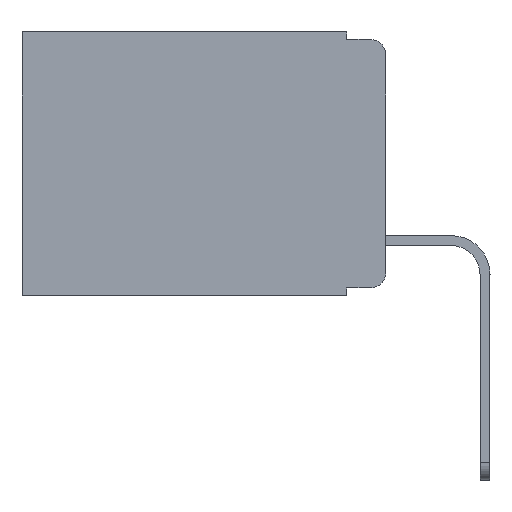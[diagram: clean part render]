
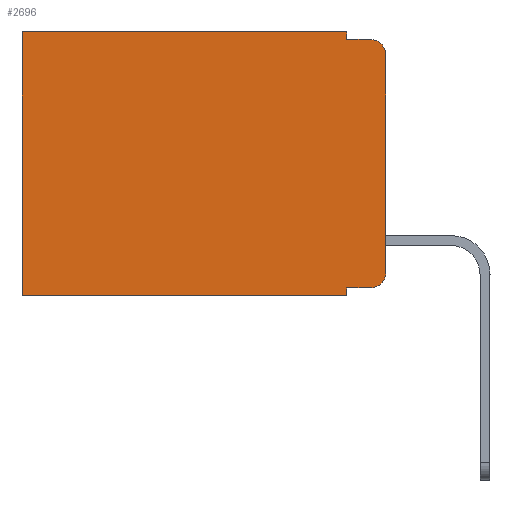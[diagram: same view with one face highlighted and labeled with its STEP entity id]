
A CAD part, left-side view. The second image highlights one B-rep face of the part: STEP entity #2696.
In plain terms, the highlighted planar face has unit normal (-1, 0, 0).
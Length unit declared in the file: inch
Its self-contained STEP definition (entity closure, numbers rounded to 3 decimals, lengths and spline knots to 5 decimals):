
#48 = CARTESIAN_POINT ( 'NONE',  ( 0.298, 0., -0.03 ) ) ;
#49 = CARTESIAN_POINT ( 'NONE',  ( 0.298, 0.051, 0. ) ) ;
#399 = DIRECTION ( 'NONE',  ( 0., 0., -1. ) ) ;
#530 = ORIENTED_EDGE ( 'NONE', *, *, #8981, .T. ) ;
#658 = VERTEX_POINT ( 'NONE', #49 ) ;
#664 = CARTESIAN_POINT ( 'NONE',  ( 0.298, 0.051, -0.333 ) ) ;
#958 = VECTOR ( 'NONE', #6136, 39.37008 ) ;
#1163 = VECTOR ( 'NONE', #10248, 39.37008 ) ;
#1909 = ORIENTED_EDGE ( 'NONE', *, *, #11181, .T. ) ;
#1912 = CARTESIAN_POINT ( 'NONE',  ( 0.298, 0.051, 0. ) ) ;
#1947 = CARTESIAN_POINT ( 'NONE',  ( 0.298, 0.473, -0.343 ) ) ;
#2083 = DIRECTION ( 'NONE',  ( -1., 0., 0. ) ) ;
#2224 = EDGE_CURVE ( 'NONE', #8301, #7767, #5740, .T. ) ;
#2696 = ADVANCED_FACE ( 'NONE', ( #5626 ), #6550, .F. ) ;
#2767 = DIRECTION ( 'NONE',  ( 0., 0., -1. ) ) ;
#3070 = VERTEX_POINT ( 'NONE', #4905 ) ;
#3289 = VECTOR ( 'NONE', #2767, 39.37008 ) ;
#3462 = ORIENTED_EDGE ( 'NONE', *, *, #12915, .F. ) ;
#3634 = EDGE_CURVE ( 'NONE', #12069, #12008, #8001, .T. ) ;
#3687 = ORIENTED_EDGE ( 'NONE', *, *, #2224, .T. ) ;
#3727 = CARTESIAN_POINT ( 'NONE',  ( 0.298, 0.02, -0.03 ) ) ;
#4110 = VECTOR ( 'NONE', #4815, 39.37008 ) ;
#4412 = AXIS2_PLACEMENT_3D ( 'NONE', #4607, #12694, #6645 ) ;
#4415 = VERTEX_POINT ( 'NONE', #11125 ) ;
#4607 = CARTESIAN_POINT ( 'NONE',  ( 0.298, 0., 0. ) ) ;
#4648 = VECTOR ( 'NONE', #10524, 39.37008 ) ;
#4815 = DIRECTION ( 'NONE',  ( 0., -1., 0. ) ) ;
#4880 = EDGE_CURVE ( 'NONE', #6598, #7418, #7479, .T. ) ;
#4905 = CARTESIAN_POINT ( 'NONE',  ( 0.298, 0.473, 0. ) ) ;
#4952 = CARTESIAN_POINT ( 'NONE',  ( 0.298, 0.051, -0.01 ) ) ;
#4972 = CARTESIAN_POINT ( 'NONE',  ( 0.298, 0.02, -0.313 ) ) ;
#5093 = CARTESIAN_POINT ( 'NONE',  ( 0.298, 0., 0. ) ) ;
#5416 = LINE ( 'NONE', #8613, #4648 ) ;
#5520 = EDGE_CURVE ( 'NONE', #4415, #7767, #12102, .T. ) ;
#5626 = FACE_OUTER_BOUND ( 'NONE', #10261, .T. ) ;
#5687 = DIRECTION ( 'NONE',  ( 0., -1., 0. ) ) ;
#5740 = CIRCLE ( 'NONE', #9652, 0.02 ) ;
#6136 = DIRECTION ( 'NONE',  ( 0., 0., -1. ) ) ;
#6403 = EDGE_CURVE ( 'NONE', #3070, #12534, #10717, .T. ) ;
#6550 = PLANE ( 'NONE',  #4412 ) ;
#6598 = VERTEX_POINT ( 'NONE', #8120 ) ;
#6645 = DIRECTION ( 'NONE',  ( 0., 0., -1. ) ) ;
#6908 = DIRECTION ( 'NONE',  ( 0., 0., -1. ) ) ;
#7068 = EDGE_CURVE ( 'NONE', #658, #4415, #9427, .T. ) ;
#7126 = ORIENTED_EDGE ( 'NONE', *, *, #6403, .T. ) ;
#7387 = LINE ( 'NONE', #664, #9278 ) ;
#7418 = VERTEX_POINT ( 'NONE', #8463 ) ;
#7479 = CIRCLE ( 'NONE', #11394, 0.02 ) ;
#7767 = VERTEX_POINT ( 'NONE', #11219 ) ;
#7928 = ORIENTED_EDGE ( 'NONE', *, *, #3634, .F. ) ;
#7990 = DIRECTION ( 'NONE',  ( 0., 0., -1. ) ) ;
#8001 = LINE ( 'NONE', #1912, #9703 ) ;
#8120 = CARTESIAN_POINT ( 'NONE',  ( 0.298, 0.02, -0.333 ) ) ;
#8221 = ORIENTED_EDGE ( 'NONE', *, *, #4880, .T. ) ;
#8301 = VERTEX_POINT ( 'NONE', #48 ) ;
#8406 = LINE ( 'NONE', #5093, #1163 ) ;
#8463 = CARTESIAN_POINT ( 'NONE',  ( 0.298, 0., -0.313 ) ) ;
#8613 = CARTESIAN_POINT ( 'NONE',  ( 0.298, 0., -0.343 ) ) ;
#8711 = ORIENTED_EDGE ( 'NONE', *, *, #5520, .F. ) ;
#8981 = EDGE_CURVE ( 'NONE', #658, #3070, #8406, .T. ) ;
#9136 = CARTESIAN_POINT ( 'NONE',  ( 0.298, 0.473, 0. ) ) ;
#9161 = CARTESIAN_POINT ( 'NONE',  ( 0.298, 0.051, -0.333 ) ) ;
#9278 = VECTOR ( 'NONE', #5687, 39.37008 ) ;
#9427 = LINE ( 'NONE', #11561, #11671 ) ;
#9652 = AXIS2_PLACEMENT_3D ( 'NONE', #3727, #12969, #6908 ) ;
#9703 = VECTOR ( 'NONE', #9965, 39.37008 ) ;
#9808 = ORIENTED_EDGE ( 'NONE', *, *, #11342, .F. ) ;
#9965 = DIRECTION ( 'NONE',  ( 0., 0., -1. ) ) ;
#10248 = DIRECTION ( 'NONE',  ( 0., 1., 0. ) ) ;
#10261 = EDGE_LOOP ( 'NONE', ( #9808, #3687, #8711, #10267, #530, #7126, #3462, #7928, #1909, #8221 ) ) ;
#10267 = ORIENTED_EDGE ( 'NONE', *, *, #7068, .F. ) ;
#10524 = DIRECTION ( 'NONE',  ( 0., 1., 0. ) ) ;
#10717 = LINE ( 'NONE', #9136, #958 ) ;
#10971 = CARTESIAN_POINT ( 'NONE',  ( 0.298, 0., 0. ) ) ;
#11125 = CARTESIAN_POINT ( 'NONE',  ( 0.298, 0.051, -0.01 ) ) ;
#11181 = EDGE_CURVE ( 'NONE', #12069, #6598, #7387, .T. ) ;
#11219 = CARTESIAN_POINT ( 'NONE',  ( 0.298, 0.02, -0.01 ) ) ;
#11342 = EDGE_CURVE ( 'NONE', #8301, #7418, #11990, .T. ) ;
#11394 = AXIS2_PLACEMENT_3D ( 'NONE', #4972, #2083, #7990 ) ;
#11561 = CARTESIAN_POINT ( 'NONE',  ( 0.298, 0.051, 0. ) ) ;
#11671 = VECTOR ( 'NONE', #399, 39.37008 ) ;
#11935 = CARTESIAN_POINT ( 'NONE',  ( 0.298, 0.051, -0.343 ) ) ;
#11990 = LINE ( 'NONE', #10971, #3289 ) ;
#12008 = VERTEX_POINT ( 'NONE', #11935 ) ;
#12069 = VERTEX_POINT ( 'NONE', #9161 ) ;
#12102 = LINE ( 'NONE', #4952, #4110 ) ;
#12534 = VERTEX_POINT ( 'NONE', #1947 ) ;
#12694 = DIRECTION ( 'NONE',  ( 1., 0., 0. ) ) ;
#12915 = EDGE_CURVE ( 'NONE', #12008, #12534, #5416, .T. ) ;
#12969 = DIRECTION ( 'NONE',  ( -1., 0., 0. ) ) ;
